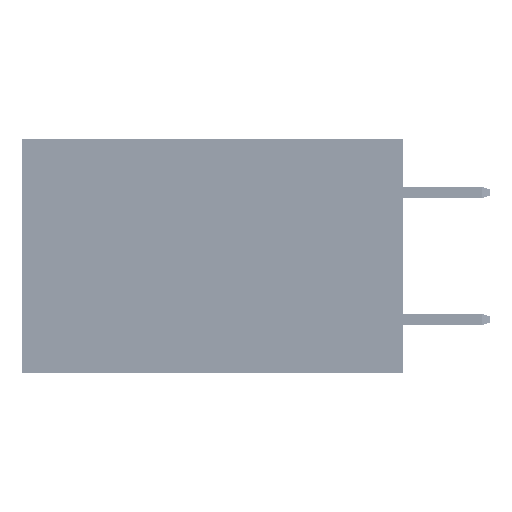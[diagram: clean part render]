
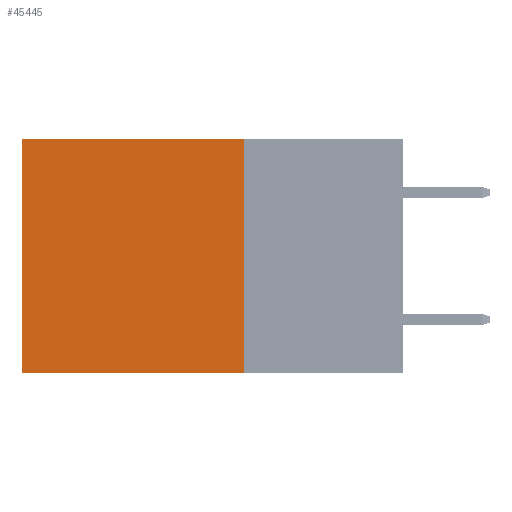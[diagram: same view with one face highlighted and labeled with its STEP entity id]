
A CAD part, left-side view. The second image highlights one B-rep face of the part: STEP entity #45445.
In plain terms, the highlighted planar face has unit normal (-1, 0, 0).
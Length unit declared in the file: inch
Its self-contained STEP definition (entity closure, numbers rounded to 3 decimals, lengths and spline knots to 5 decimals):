
#838 = CARTESIAN_POINT ( 'NONE',  ( 0.2875, 0.25, 0. ) ) ;
#1281 = LINE ( 'NONE', #30960, #21453 ) ;
#2082 = VECTOR ( 'NONE', #37397, 39.37008 ) ;
#3256 = EDGE_CURVE ( 'NONE', #26277, #25774, #1281, .T. ) ;
#5461 = DIRECTION ( 'NONE',  ( 1., 0., 0. ) ) ;
#6996 = EDGE_CURVE ( 'NONE', #17218, #25774, #30387, .T. ) ;
#7976 = DIRECTION ( 'NONE',  ( 0., 1., 0. ) ) ;
#10472 = AXIS2_PLACEMENT_3D ( 'NONE', #46807, #5461, #33768 ) ;
#13067 = EDGE_CURVE ( 'NONE', #33699, #26277, #20820, .T. ) ;
#17218 = VERTEX_POINT ( 'NONE', #33306 ) ;
#17286 = VECTOR ( 'NONE', #42354, 39.37008 ) ;
#18263 = VECTOR ( 'NONE', #7976, 39.37008 ) ;
#20820 = LINE ( 'NONE', #50722, #2082 ) ;
#21453 = VECTOR ( 'NONE', #22536, 39.37008 ) ;
#22536 = DIRECTION ( 'NONE',  ( 0., 1., 0. ) ) ;
#25774 = VERTEX_POINT ( 'NONE', #51511 ) ;
#25987 = ORIENTED_EDGE ( 'NONE', *, *, #13067, .F. ) ;
#26277 = VERTEX_POINT ( 'NONE', #39459 ) ;
#27491 = EDGE_CURVE ( 'NONE', #33699, #17218, #53152, .T. ) ;
#30387 = LINE ( 'NONE', #38261, #17286 ) ;
#30960 = CARTESIAN_POINT ( 'NONE',  ( 0.2875, 0.25, -0.37 ) ) ;
#32371 = EDGE_LOOP ( 'NONE', ( #41118, #51721, #25987, #52250 ) ) ;
#32465 = CARTESIAN_POINT ( 'NONE',  ( 0.2875, 0.25, 0. ) ) ;
#33306 = CARTESIAN_POINT ( 'NONE',  ( 0.2875, 0.6, 0. ) ) ;
#33699 = VERTEX_POINT ( 'NONE', #838 ) ;
#33768 = DIRECTION ( 'NONE',  ( 0., 0., -1. ) ) ;
#37397 = DIRECTION ( 'NONE',  ( 0., 0., -1. ) ) ;
#38261 = CARTESIAN_POINT ( 'NONE',  ( 0.2875, 0.6, 0. ) ) ;
#39459 = CARTESIAN_POINT ( 'NONE',  ( 0.2875, 0.25, -0.37 ) ) ;
#41118 = ORIENTED_EDGE ( 'NONE', *, *, #6996, .T. ) ;
#41927 = PLANE ( 'NONE',  #10472 ) ;
#42354 = DIRECTION ( 'NONE',  ( 0., 0., -1. ) ) ;
#45445 = ADVANCED_FACE ( 'NONE', ( #47065 ), #41927, .F. ) ;
#46807 = CARTESIAN_POINT ( 'NONE',  ( 0.2875, 0.25, 0. ) ) ;
#47065 = FACE_OUTER_BOUND ( 'NONE', #32371, .T. ) ;
#50722 = CARTESIAN_POINT ( 'NONE',  ( 0.2875, 0.25, 0. ) ) ;
#51511 = CARTESIAN_POINT ( 'NONE',  ( 0.2875, 0.6, -0.37 ) ) ;
#51721 = ORIENTED_EDGE ( 'NONE', *, *, #3256, .F. ) ;
#52250 = ORIENTED_EDGE ( 'NONE', *, *, #27491, .T. ) ;
#53152 = LINE ( 'NONE', #32465, #18263 ) ;
